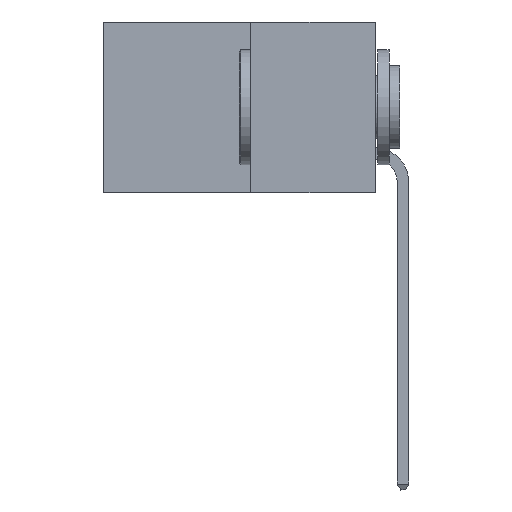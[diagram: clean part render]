
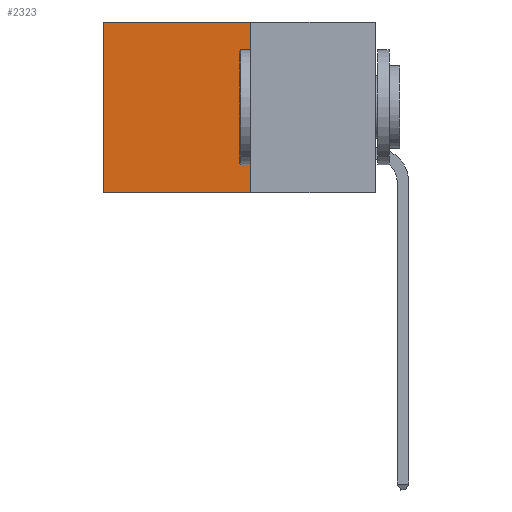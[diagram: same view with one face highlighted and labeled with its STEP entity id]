
A CAD part, left-side view. The second image highlights one B-rep face of the part: STEP entity #2323.
In plain terms, the highlighted planar face has unit normal (-1, 0, 0).
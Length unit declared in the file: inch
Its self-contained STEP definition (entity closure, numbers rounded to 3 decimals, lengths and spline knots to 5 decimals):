
#141 = DIRECTION ( 'NONE',  ( 0., 1., 0. ) ) ;
#445 = ORIENTED_EDGE ( 'NONE', *, *, #10611, .F. ) ;
#689 = DIRECTION ( 'NONE',  ( 0., 0., -1. ) ) ;
#763 = ORIENTED_EDGE ( 'NONE', *, *, #6740, .F. ) ;
#1111 = EDGE_CURVE ( 'NONE', #6220, #5238, #3302, .T. ) ;
#1670 = VECTOR ( 'NONE', #689, 39.37008 ) ;
#1990 = LINE ( 'NONE', #4802, #12035 ) ;
#2323 = ADVANCED_FACE ( 'NONE', ( #8245 ), #9364, .F. ) ;
#2417 = CARTESIAN_POINT ( 'NONE',  ( 0.277, 0.59, -0.37 ) ) ;
#2558 = ORIENTED_EDGE ( 'NONE', *, *, #6758, .T. ) ;
#2683 = CARTESIAN_POINT ( 'NONE',  ( 0.277, 0.59, 0. ) ) ;
#3302 = LINE ( 'NONE', #6655, #8412 ) ;
#3779 = CARTESIAN_POINT ( 'NONE',  ( 0.277, 0.27, -0.37 ) ) ;
#3827 = DIRECTION ( 'NONE',  ( 0., 0., -1. ) ) ;
#4391 = LINE ( 'NONE', #3779, #1670 ) ;
#4784 = AXIS2_PLACEMENT_3D ( 'NONE', #9746, #9226, #9209 ) ;
#4802 = CARTESIAN_POINT ( 'NONE',  ( 0.277, 0.27, -0.37 ) ) ;
#5238 = VERTEX_POINT ( 'NONE', #2683 ) ;
#6220 = VERTEX_POINT ( 'NONE', #7039 ) ;
#6350 = EDGE_LOOP ( 'NONE', ( #2558, #445, #763, #7301 ) ) ;
#6655 = CARTESIAN_POINT ( 'NONE',  ( 0.277, 0.27, 0. ) ) ;
#6740 = EDGE_CURVE ( 'NONE', #6220, #8047, #4391, .T. ) ;
#6758 = EDGE_CURVE ( 'NONE', #5238, #7354, #6766, .T. ) ;
#6766 = LINE ( 'NONE', #7640, #11539 ) ;
#7039 = CARTESIAN_POINT ( 'NONE',  ( 0.277, 0.27, 0. ) ) ;
#7301 = ORIENTED_EDGE ( 'NONE', *, *, #1111, .T. ) ;
#7354 = VERTEX_POINT ( 'NONE', #2417 ) ;
#7640 = CARTESIAN_POINT ( 'NONE',  ( 0.277, 0.59, -0.37 ) ) ;
#8047 = VERTEX_POINT ( 'NONE', #11981 ) ;
#8245 = FACE_OUTER_BOUND ( 'NONE', #6350, .T. ) ;
#8412 = VECTOR ( 'NONE', #141, 39.37008 ) ;
#9209 = DIRECTION ( 'NONE',  ( 0., 0., -1. ) ) ;
#9226 = DIRECTION ( 'NONE',  ( 1., 0., 0. ) ) ;
#9364 = PLANE ( 'NONE',  #4784 ) ;
#9560 = DIRECTION ( 'NONE',  ( 0., 1., 0. ) ) ;
#9746 = CARTESIAN_POINT ( 'NONE',  ( 0.277, 0.27, -0.37 ) ) ;
#10611 = EDGE_CURVE ( 'NONE', #8047, #7354, #1990, .T. ) ;
#11539 = VECTOR ( 'NONE', #3827, 39.37008 ) ;
#11981 = CARTESIAN_POINT ( 'NONE',  ( 0.277, 0.27, -0.37 ) ) ;
#12035 = VECTOR ( 'NONE', #9560, 39.37008 ) ;
